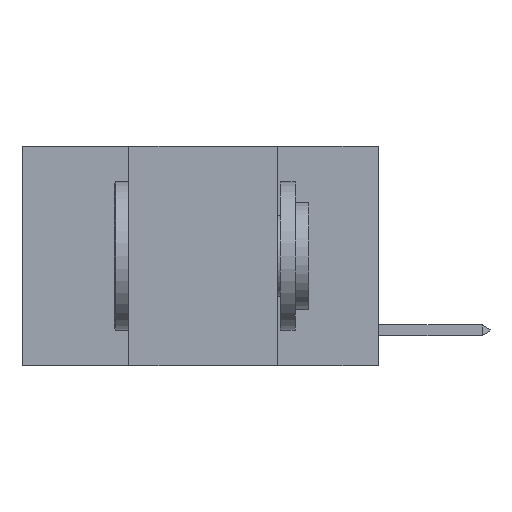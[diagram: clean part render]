
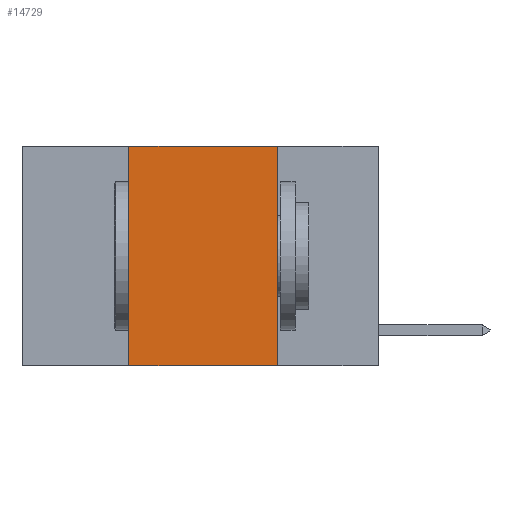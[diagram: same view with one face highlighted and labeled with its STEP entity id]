
A CAD part, left-side view. The second image highlights one B-rep face of the part: STEP entity #14729.
In plain terms, the highlighted planar face has unit normal (-1, 0, 0).
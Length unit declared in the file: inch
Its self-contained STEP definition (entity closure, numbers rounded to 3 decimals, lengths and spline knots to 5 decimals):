
#136 = EDGE_CURVE ( 'NONE', #6426, #6019, #14514, .T. ) ;
#158 = EDGE_LOOP ( 'NONE', ( #2156, #20114, #14375, #4525 ) ) ;
#1262 = CARTESIAN_POINT ( 'NONE',  ( 0., 0.17, -0.37 ) ) ;
#1520 = VECTOR ( 'NONE', #12387, 39.37008 ) ;
#2156 = ORIENTED_EDGE ( 'NONE', *, *, #9904, .F. ) ;
#2304 = VECTOR ( 'NONE', #20514, 39.37008 ) ;
#2842 = AXIS2_PLACEMENT_3D ( 'NONE', #3687, #9141, #21557 ) ;
#3687 = CARTESIAN_POINT ( 'NONE',  ( 0., 0.6, 0. ) ) ;
#4155 = FACE_OUTER_BOUND ( 'NONE', #158, .T. ) ;
#4525 = ORIENTED_EDGE ( 'NONE', *, *, #18633, .T. ) ;
#4939 = VECTOR ( 'NONE', #19765, 39.37008 ) ;
#5080 = VERTEX_POINT ( 'NONE', #1262 ) ;
#5734 = LINE ( 'NONE', #22916, #1520 ) ;
#6019 = VERTEX_POINT ( 'NONE', #17282 ) ;
#6426 = VERTEX_POINT ( 'NONE', #20127 ) ;
#7252 = CARTESIAN_POINT ( 'NONE',  ( 0., 0.17, 0. ) ) ;
#7311 = PLANE ( 'NONE',  #2842 ) ;
#9141 = DIRECTION ( 'NONE',  ( 1., 0., 0. ) ) ;
#9904 = EDGE_CURVE ( 'NONE', #12115, #5080, #18692, .T. ) ;
#11324 = EDGE_CURVE ( 'NONE', #6019, #12115, #5734, .T. ) ;
#11339 = CARTESIAN_POINT ( 'NONE',  ( 0., 0.42, 0. ) ) ;
#11600 = DIRECTION ( 'NONE',  ( 0., 0., 1. ) ) ;
#12115 = VERTEX_POINT ( 'NONE', #18084 ) ;
#12387 = DIRECTION ( 'NONE',  ( 0., -1., 0. ) ) ;
#14375 = ORIENTED_EDGE ( 'NONE', *, *, #136, .F. ) ;
#14514 = LINE ( 'NONE', #11339, #18688 ) ;
#14729 = ADVANCED_FACE ( 'NONE', ( #4155 ), #7311, .F. ) ;
#16648 = LINE ( 'NONE', #18750, #2304 ) ;
#17282 = CARTESIAN_POINT ( 'NONE',  ( 0., 0.42, 0. ) ) ;
#18084 = CARTESIAN_POINT ( 'NONE',  ( 0., 0.17, 0. ) ) ;
#18633 = EDGE_CURVE ( 'NONE', #6426, #5080, #16648, .T. ) ;
#18688 = VECTOR ( 'NONE', #11600, 39.37008 ) ;
#18692 = LINE ( 'NONE', #7252, #4939 ) ;
#18750 = CARTESIAN_POINT ( 'NONE',  ( 0., 0.6, -0.37 ) ) ;
#19765 = DIRECTION ( 'NONE',  ( 0., 0., -1. ) ) ;
#20114 = ORIENTED_EDGE ( 'NONE', *, *, #11324, .F. ) ;
#20127 = CARTESIAN_POINT ( 'NONE',  ( 0., 0.42, -0.37 ) ) ;
#20514 = DIRECTION ( 'NONE',  ( 0., -1., 0. ) ) ;
#21557 = DIRECTION ( 'NONE',  ( 0., 0., -1. ) ) ;
#22916 = CARTESIAN_POINT ( 'NONE',  ( 0., 0.6, 0. ) ) ;
